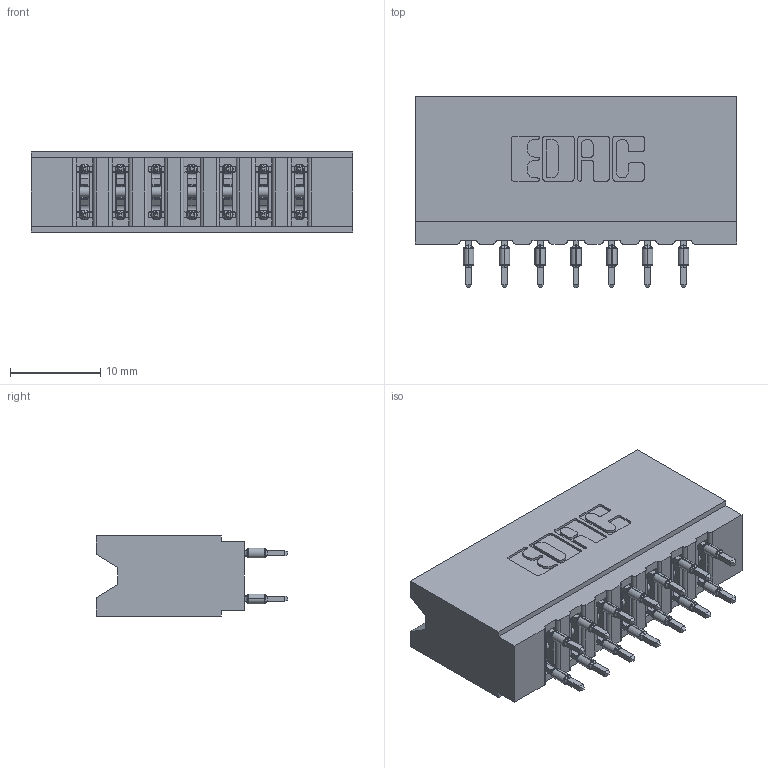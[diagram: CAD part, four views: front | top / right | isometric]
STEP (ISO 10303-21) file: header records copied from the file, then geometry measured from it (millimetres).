
FILE_DESCRIPTION (( 'STEP AP203' ), '1' );
FILE_NAME ('737-014-560-206.STEP', '2026-03-05T21:19:51', ( '' ), ( '' ), 'SwSTEP 2.0', 'SolidWorks 2023', '' );
FILE_SCHEMA (( 'CONFIG_CONTROL_DESIGN' ));
Length unit declared in the file: millimetre
Products named in the file (3): 737-014-560-206; 745-292-001_560; 737 Part_Insulator Option - 06
Assembly tree (15 placements, depth 2):
  737-014-560-206
    737 Part_Insulator Option - 06
    745-292-001_560  x14
Bounding box: 35.61 x 21.22 x 8.89 mm (x, y, z)
Volume: 3712.8 mm3; surface area: 5236.6 mm2
Topology: 15 solids, 15 shells, 1481 faces, 4051 edges, 2578 vertices
Faces by surface type: plane 776, cylinder 341, bspline 280, torus 84
Entity records: 17104 total; most frequent: CARTESIAN_POINT 3484, ORIENTED_EDGE 2850, DIRECTION 2523, EDGE_CURVE 1425, LINE 1193, VECTOR 1193, VERTEX_POINT 914, AXIS2_PLACEMENT_3D 665
